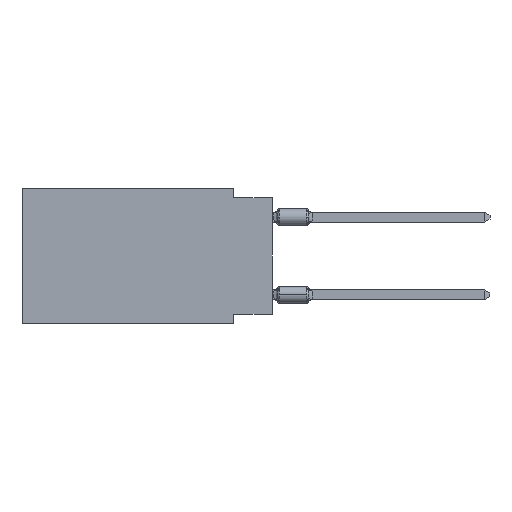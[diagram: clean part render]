
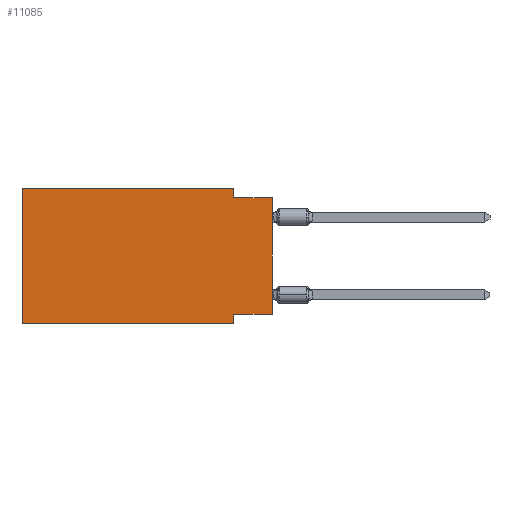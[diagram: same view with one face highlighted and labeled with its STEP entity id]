
A CAD part, left-side view. The second image highlights one B-rep face of the part: STEP entity #11085.
In plain terms, the highlighted planar face has unit normal (-1, 0, 0).
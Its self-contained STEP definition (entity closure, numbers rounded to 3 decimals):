
#303 = VECTOR ( 'NONE', #9134, 1000. ) ;
#545 = DIRECTION ( 'NONE',  ( 0., -1., 0. ) ) ;
#701 = EDGE_CURVE ( 'NONE', #6906, #2611, #3445, .T. ) ;
#756 = EDGE_CURVE ( 'NONE', #9801, #1894, #12622, .T. ) ;
#985 = CARTESIAN_POINT ( 'NONE',  ( 0., 2.54, -8.89 ) ) ;
#1056 = VERTEX_POINT ( 'NONE', #2029 ) ;
#1102 = ORIENTED_EDGE ( 'NONE', *, *, #12979, .F. ) ;
#1763 = LINE ( 'NONE', #7430, #4692 ) ;
#1878 = CARTESIAN_POINT ( 'NONE',  ( 0., 0., -8.255 ) ) ;
#1894 = VERTEX_POINT ( 'NONE', #8953 ) ;
#1936 = ORIENTED_EDGE ( 'NONE', *, *, #15711, .F. ) ;
#2029 = CARTESIAN_POINT ( 'NONE',  ( 0., 0., -0.635 ) ) ;
#2046 = CARTESIAN_POINT ( 'NONE',  ( 0., 2.54, 0. ) ) ;
#2611 = VERTEX_POINT ( 'NONE', #10673 ) ;
#2682 = ORIENTED_EDGE ( 'NONE', *, *, #3484, .F. ) ;
#3445 = LINE ( 'NONE', #2046, #3916 ) ;
#3484 = EDGE_CURVE ( 'NONE', #2611, #1056, #16274, .T. ) ;
#3822 = EDGE_CURVE ( 'NONE', #9801, #9955, #15206, .T. ) ;
#3871 = DIRECTION ( 'NONE',  ( 0., 0., -1. ) ) ;
#3916 = VECTOR ( 'NONE', #10594, 1000. ) ;
#4547 = AXIS2_PLACEMENT_3D ( 'NONE', #10898, #17674, #7922 ) ;
#4692 = VECTOR ( 'NONE', #545, 1000. ) ;
#4716 = EDGE_LOOP ( 'NONE', ( #5272, #2682, #12027, #1102, #11927, #15133, #1936, #18206 ) ) ;
#4934 = DIRECTION ( 'NONE',  ( 0., 0., 1. ) ) ;
#5272 = ORIENTED_EDGE ( 'NONE', *, *, #7219, .T. ) ;
#5565 = DIRECTION ( 'NONE',  ( 0., -1., 0. ) ) ;
#5920 = VECTOR ( 'NONE', #4934, 1000. ) ;
#6855 = DIRECTION ( 'NONE',  ( 0., 0., 1. ) ) ;
#6906 = VERTEX_POINT ( 'NONE', #9489 ) ;
#7219 = EDGE_CURVE ( 'NONE', #14705, #1056, #11620, .T. ) ;
#7430 = CARTESIAN_POINT ( 'NONE',  ( 0., 16.383, 0. ) ) ;
#7572 = CARTESIAN_POINT ( 'NONE',  ( 0., 0., -8.255 ) ) ;
#7813 = VECTOR ( 'NONE', #5565, 1000. ) ;
#7922 = DIRECTION ( 'NONE',  ( 0., 0., -1. ) ) ;
#8119 = VECTOR ( 'NONE', #3871, 1000. ) ;
#8248 = CARTESIAN_POINT ( 'NONE',  ( 0., 16.383, 0. ) ) ;
#8953 = CARTESIAN_POINT ( 'NONE',  ( 0., 2.54, -8.89 ) ) ;
#9134 = DIRECTION ( 'NONE',  ( 0., -1., 0. ) ) ;
#9305 = FACE_OUTER_BOUND ( 'NONE', #4716, .T. ) ;
#9489 = CARTESIAN_POINT ( 'NONE',  ( 0., 2.54, 0. ) ) ;
#9588 = PLANE ( 'NONE',  #4547 ) ;
#9675 = VECTOR ( 'NONE', #6855, 1000. ) ;
#9711 = VECTOR ( 'NONE', #16084, 1000. ) ;
#9801 = VERTEX_POINT ( 'NONE', #15584 ) ;
#9955 = VERTEX_POINT ( 'NONE', #17892 ) ;
#10594 = DIRECTION ( 'NONE',  ( 0., 0., -1. ) ) ;
#10673 = CARTESIAN_POINT ( 'NONE',  ( 0., 2.54, -0.635 ) ) ;
#10898 = CARTESIAN_POINT ( 'NONE',  ( 0., 16.383, 0. ) ) ;
#10902 = CARTESIAN_POINT ( 'NONE',  ( 0., 0., -0.635 ) ) ;
#11085 = ADVANCED_FACE ( 'NONE', ( #9305 ), #9588, .F. ) ;
#11620 = LINE ( 'NONE', #11991, #5920 ) ;
#11927 = ORIENTED_EDGE ( 'NONE', *, *, #3822, .F. ) ;
#11991 = CARTESIAN_POINT ( 'NONE',  ( 0., 0., 0. ) ) ;
#12027 = ORIENTED_EDGE ( 'NONE', *, *, #701, .F. ) ;
#12458 = EDGE_CURVE ( 'NONE', #14705, #15845, #14505, .T. ) ;
#12622 = LINE ( 'NONE', #18282, #7813 ) ;
#12965 = CARTESIAN_POINT ( 'NONE',  ( 0., 2.54, -8.255 ) ) ;
#12979 = EDGE_CURVE ( 'NONE', #9955, #6906, #1763, .T. ) ;
#14505 = LINE ( 'NONE', #1878, #9711 ) ;
#14705 = VERTEX_POINT ( 'NONE', #7572 ) ;
#15093 = LINE ( 'NONE', #985, #8119 ) ;
#15133 = ORIENTED_EDGE ( 'NONE', *, *, #756, .T. ) ;
#15206 = LINE ( 'NONE', #8248, #9675 ) ;
#15584 = CARTESIAN_POINT ( 'NONE',  ( 0., 16.383, -8.89 ) ) ;
#15711 = EDGE_CURVE ( 'NONE', #15845, #1894, #15093, .T. ) ;
#15845 = VERTEX_POINT ( 'NONE', #12965 ) ;
#16084 = DIRECTION ( 'NONE',  ( 0., 1., 0. ) ) ;
#16274 = LINE ( 'NONE', #10902, #303 ) ;
#17674 = DIRECTION ( 'NONE',  ( 1., 0., 0. ) ) ;
#17892 = CARTESIAN_POINT ( 'NONE',  ( 0., 16.383, 0. ) ) ;
#18206 = ORIENTED_EDGE ( 'NONE', *, *, #12458, .F. ) ;
#18282 = CARTESIAN_POINT ( 'NONE',  ( 0., 16.383, -8.89 ) ) ;
